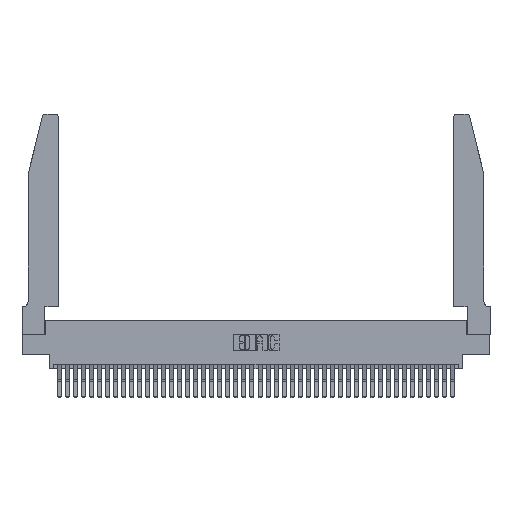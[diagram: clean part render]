
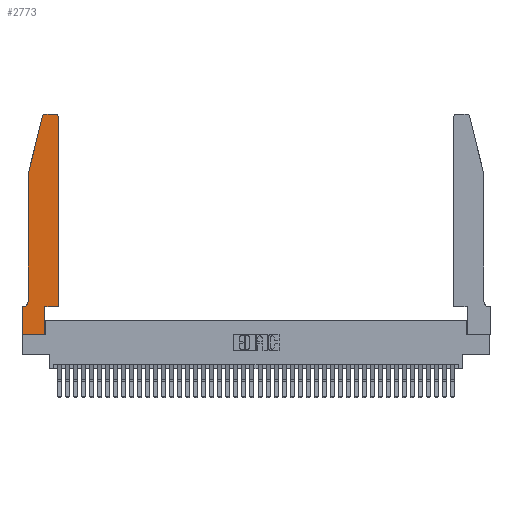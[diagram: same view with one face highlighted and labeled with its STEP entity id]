
A CAD part, top view. The second image highlights one B-rep face of the part: STEP entity #2773.
In plain terms, the highlighted planar face has unit normal (0, 0, 1).
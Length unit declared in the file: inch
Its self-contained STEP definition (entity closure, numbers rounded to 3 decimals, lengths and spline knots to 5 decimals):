
#507 = LINE ( 'NONE', #15746, #17438 ) ;
#829 = VECTOR ( 'NONE', #9043, 39.37008 ) ;
#1238 = EDGE_CURVE ( 'NONE', #8358, #10733, #29183, .T. ) ;
#1541 = ORIENTED_EDGE ( 'NONE', *, *, #22272, .T. ) ;
#1620 = CARTESIAN_POINT ( 'NONE',  ( 0.0055, 0.42, 0.37 ) ) ;
#1872 = EDGE_CURVE ( 'NONE', #22810, #10324, #26061, .T. ) ;
#2025 = EDGE_CURVE ( 'NONE', #3218, #7502, #19861, .T. ) ;
#2544 = LINE ( 'NONE', #16457, #10497 ) ;
#2773 = ADVANCED_FACE ( 'NONE', ( #9891 ), #9724, .T. ) ;
#2899 = DIRECTION ( 'NONE',  ( 0., -1., 0. ) ) ;
#3218 = VERTEX_POINT ( 'NONE', #38382 ) ;
#3652 = ORIENTED_EDGE ( 'NONE', *, *, #38443, .T. ) ;
#3965 = ORIENTED_EDGE ( 'NONE', *, *, #2025, .T. ) ;
#4731 = DIRECTION ( 'NONE',  ( -1., 0., 0. ) ) ;
#5090 = DIRECTION ( 'NONE',  ( -1., 0., 0. ) ) ;
#5673 = CARTESIAN_POINT ( 'NONE',  ( 0.4505, 0.35, 0.37 ) ) ;
#6025 = ORIENTED_EDGE ( 'NONE', *, *, #24313, .T. ) ;
#6153 = EDGE_CURVE ( 'NONE', #8850, #27432, #2544, .T. ) ;
#6459 = LINE ( 'NONE', #20218, #40691 ) ;
#7274 = CARTESIAN_POINT ( 'NONE',  ( 0.2865, 0.35, 0.37 ) ) ;
#7341 = DIRECTION ( 'NONE',  ( 0., 0., 1. ) ) ;
#7446 = CARTESIAN_POINT ( 'NONE',  ( 0.2865, 0., 0.37 ) ) ;
#7502 = VERTEX_POINT ( 'NONE', #28641 ) ;
#8358 = VERTEX_POINT ( 'NONE', #35778 ) ;
#8580 = ORIENTED_EDGE ( 'NONE', *, *, #1238, .T. ) ;
#8850 = VERTEX_POINT ( 'NONE', #5673 ) ;
#9043 = DIRECTION ( 'NONE',  ( -1., 0., 0. ) ) ;
#9188 = VECTOR ( 'NONE', #13140, 39.37008 ) ;
#9302 = VECTOR ( 'NONE', #4731, 39.37008 ) ;
#9724 = PLANE ( 'NONE',  #29497 ) ;
#9891 = FACE_OUTER_BOUND ( 'NONE', #14241, .T. ) ;
#10324 = VERTEX_POINT ( 'NONE', #35450 ) ;
#10497 = VECTOR ( 'NONE', #39559, 39.37008 ) ;
#10733 = VERTEX_POINT ( 'NONE', #7446 ) ;
#10964 = EDGE_CURVE ( 'NONE', #41446, #8850, #507, .T. ) ;
#11494 = VECTOR ( 'NONE', #34770, 39.37008 ) ;
#11949 = CIRCLE ( 'NONE', #34984, 0.03 ) ;
#12373 = DIRECTION ( 'NONE',  ( 1., 0., 0. ) ) ;
#12402 = CARTESIAN_POINT ( 'NONE',  ( 0.2605, 2.75, 0.37 ) ) ;
#12838 = ORIENTED_EDGE ( 'NONE', *, *, #41285, .T. ) ;
#13140 = DIRECTION ( 'NONE',  ( 0., -1., 0. ) ) ;
#13216 = EDGE_CURVE ( 'NONE', #7502, #15861, #11949, .T. ) ;
#14241 = EDGE_LOOP ( 'NONE', ( #3965, #28881, #1541, #6025, #15054, #18576, #12838, #8580, #34696, #24236, #36962, #3652 ) ) ;
#15054 = ORIENTED_EDGE ( 'NONE', *, *, #1872, .T. ) ;
#15746 = CARTESIAN_POINT ( 'NONE',  ( 0.4505, 0.35, 0.37 ) ) ;
#15861 = VERTEX_POINT ( 'NONE', #19370 ) ;
#16455 = DIRECTION ( 'NONE',  ( 1., 0., 0. ) ) ;
#16457 = CARTESIAN_POINT ( 'NONE',  ( 0.4505, 0.35, 0.37 ) ) ;
#17438 = VECTOR ( 'NONE', #12373, 39.37008 ) ;
#18048 = EDGE_CURVE ( 'NONE', #10733, #41446, #6459, .T. ) ;
#18134 = LINE ( 'NONE', #29676, #9188 ) ;
#18576 = ORIENTED_EDGE ( 'NONE', *, *, #31764, .T. ) ;
#19116 = CARTESIAN_POINT ( 'NONE',  ( 0.4205, 2.72, 0.37 ) ) ;
#19316 = VERTEX_POINT ( 'NONE', #21263 ) ;
#19370 = CARTESIAN_POINT ( 'NONE',  ( 0.25487, 2.72718, 0.37 ) ) ;
#19861 = LINE ( 'NONE', #12402, #829 ) ;
#20218 = CARTESIAN_POINT ( 'NONE',  ( 0.2865, 0.35, 0.37 ) ) ;
#20346 = LINE ( 'NONE', #21446, #9302 ) ;
#21263 = CARTESIAN_POINT ( 'NONE',  ( 0.0755, 2., 0.37 ) ) ;
#21446 = CARTESIAN_POINT ( 'NONE',  ( 0.0755, 0.35, 0.37 ) ) ;
#22272 = EDGE_CURVE ( 'NONE', #15861, #19316, #23450, .T. ) ;
#22463 = DIRECTION ( 'NONE',  ( 1., 0., 0. ) ) ;
#22810 = VERTEX_POINT ( 'NONE', #25157 ) ;
#23039 = CARTESIAN_POINT ( 'NONE',  ( 0.0755, 2., 0.37 ) ) ;
#23450 = LINE ( 'NONE', #42320, #39886 ) ;
#24236 = ORIENTED_EDGE ( 'NONE', *, *, #10964, .T. ) ;
#24313 = EDGE_CURVE ( 'NONE', #19316, #22810, #41255, .T. ) ;
#25114 = DIRECTION ( 'NONE',  ( 0., 0., -1. ) ) ;
#25157 = CARTESIAN_POINT ( 'NONE',  ( 0.0755, 0.42, 0.37 ) ) ;
#25848 = CARTESIAN_POINT ( 'NONE',  ( 0., 0.35, 0.37 ) ) ;
#25904 = DIRECTION ( 'NONE',  ( -0.239, -0.971, 0. ) ) ;
#26061 = CIRCLE ( 'NONE', #36372, 0.07 ) ;
#26860 = DIRECTION ( 'NONE',  ( 0., 1., 0. ) ) ;
#27288 = CARTESIAN_POINT ( 'NONE',  ( 0.284, 2.72, 0.37 ) ) ;
#27432 = VERTEX_POINT ( 'NONE', #36267 ) ;
#28641 = CARTESIAN_POINT ( 'NONE',  ( 0.284, 2.75, 0.37 ) ) ;
#28881 = ORIENTED_EDGE ( 'NONE', *, *, #13216, .T. ) ;
#29183 = LINE ( 'NONE', #38094, #11494 ) ;
#29497 = AXIS2_PLACEMENT_3D ( 'NONE', #32942, #36242, #16455 ) ;
#29676 = CARTESIAN_POINT ( 'NONE',  ( 0., 0., 0.37 ) ) ;
#30595 = DIRECTION ( 'NONE',  ( 1., 0., 0. ) ) ;
#30712 = CIRCLE ( 'NONE', #36606, 0.03 ) ;
#31764 = EDGE_CURVE ( 'NONE', #10324, #39092, #20346, .T. ) ;
#32942 = CARTESIAN_POINT ( 'NONE',  ( 0., 0.35, 0.37 ) ) ;
#34696 = ORIENTED_EDGE ( 'NONE', *, *, #18048, .T. ) ;
#34770 = DIRECTION ( 'NONE',  ( 1., 0., 0. ) ) ;
#34984 = AXIS2_PLACEMENT_3D ( 'NONE', #27288, #7341, #30595 ) ;
#35450 = CARTESIAN_POINT ( 'NONE',  ( 0.0055, 0.35, 0.37 ) ) ;
#35778 = CARTESIAN_POINT ( 'NONE',  ( 0., 0., 0.37 ) ) ;
#36242 = DIRECTION ( 'NONE',  ( 0., 0., 1. ) ) ;
#36267 = CARTESIAN_POINT ( 'NONE',  ( 0.4505, 2.72, 0.37 ) ) ;
#36372 = AXIS2_PLACEMENT_3D ( 'NONE', #1620, #25114, #5090 ) ;
#36606 = AXIS2_PLACEMENT_3D ( 'NONE', #19116, #42173, #22463 ) ;
#36962 = ORIENTED_EDGE ( 'NONE', *, *, #6153, .T. ) ;
#38094 = CARTESIAN_POINT ( 'NONE',  ( 0., 0., 0.37 ) ) ;
#38382 = CARTESIAN_POINT ( 'NONE',  ( 0.4205, 2.75, 0.37 ) ) ;
#38443 = EDGE_CURVE ( 'NONE', #27432, #3218, #30712, .T. ) ;
#39092 = VERTEX_POINT ( 'NONE', #25848 ) ;
#39559 = DIRECTION ( 'NONE',  ( 0., 1., 0. ) ) ;
#39886 = VECTOR ( 'NONE', #25904, 39.37008 ) ;
#40221 = VECTOR ( 'NONE', #2899, 39.37008 ) ;
#40691 = VECTOR ( 'NONE', #26860, 39.37008 ) ;
#41255 = LINE ( 'NONE', #23039, #40221 ) ;
#41285 = EDGE_CURVE ( 'NONE', #39092, #8358, #18134, .T. ) ;
#41446 = VERTEX_POINT ( 'NONE', #7274 ) ;
#42173 = DIRECTION ( 'NONE',  ( 0., 0., 1. ) ) ;
#42320 = CARTESIAN_POINT ( 'NONE',  ( 0.0755, 2., 0.37 ) ) ;
